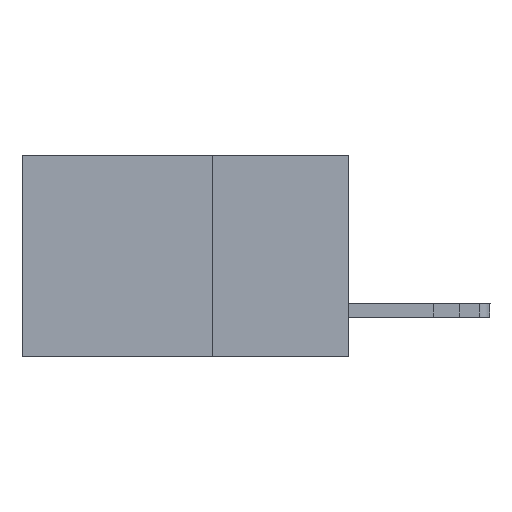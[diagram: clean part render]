
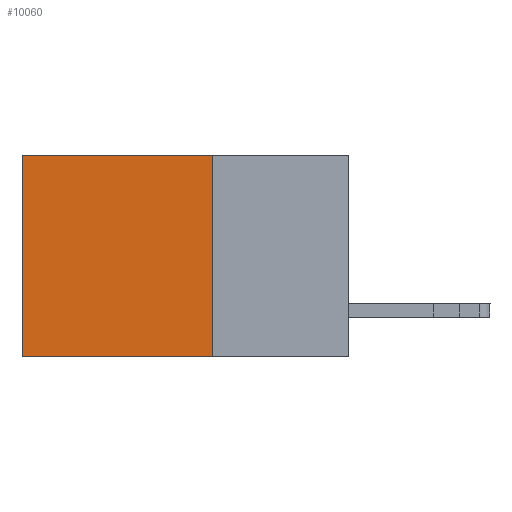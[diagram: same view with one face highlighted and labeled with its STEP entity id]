
A CAD part, left-side view. The second image highlights one B-rep face of the part: STEP entity #10060.
In plain terms, the highlighted planar face has unit normal (-1, 0, 0).
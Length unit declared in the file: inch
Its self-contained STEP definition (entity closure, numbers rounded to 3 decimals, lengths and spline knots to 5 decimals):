
#1041 = ORIENTED_EDGE ( 'NONE', *, *, #10979, .T. ) ;
#1386 = CARTESIAN_POINT ( 'NONE',  ( 0.298, 0.25, 0. ) ) ;
#1926 = CARTESIAN_POINT ( 'NONE',  ( 0.298, 0.25, 0. ) ) ;
#1975 = CARTESIAN_POINT ( 'NONE',  ( 0.298, 0.6, -0.37 ) ) ;
#2164 = CARTESIAN_POINT ( 'NONE',  ( 0.298, 0.25, 0. ) ) ;
#2579 = CARTESIAN_POINT ( 'NONE',  ( 0.298, 0.25, -0.37 ) ) ;
#2600 = CARTESIAN_POINT ( 'NONE',  ( 0.298, 0.6, 0. ) ) ;
#2661 = ORIENTED_EDGE ( 'NONE', *, *, #10180, .F. ) ;
#2903 = ORIENTED_EDGE ( 'NONE', *, *, #3127, .T. ) ;
#2973 = ORIENTED_EDGE ( 'NONE', *, *, #8306, .F. ) ;
#3000 = VECTOR ( 'NONE', #5588, 39.37008 ) ;
#3127 = EDGE_CURVE ( 'NONE', #6355, #10970, #6141, .T. ) ;
#3962 = VECTOR ( 'NONE', #13827, 39.37008 ) ;
#4006 = LINE ( 'NONE', #1386, #9899 ) ;
#4305 = CARTESIAN_POINT ( 'NONE',  ( 0.298, 0.25, -0.37 ) ) ;
#5404 = DIRECTION ( 'NONE',  ( 1., 0., 0. ) ) ;
#5450 = CARTESIAN_POINT ( 'NONE',  ( 0.298, 0.25, 0. ) ) ;
#5588 = DIRECTION ( 'NONE',  ( 0., 1., 0. ) ) ;
#5923 = VERTEX_POINT ( 'NONE', #1975 ) ;
#6002 = LINE ( 'NONE', #4305, #3962 ) ;
#6017 = FACE_OUTER_BOUND ( 'NONE', #13135, .T. ) ;
#6141 = LINE ( 'NONE', #2164, #3000 ) ;
#6233 = DIRECTION ( 'NONE',  ( 0., 0., -1. ) ) ;
#6355 = VERTEX_POINT ( 'NONE', #1926 ) ;
#7403 = CARTESIAN_POINT ( 'NONE',  ( 0.298, 0.6, 0. ) ) ;
#7746 = PLANE ( 'NONE',  #8399 ) ;
#8158 = LINE ( 'NONE', #7403, #8531 ) ;
#8306 = EDGE_CURVE ( 'NONE', #6355, #12272, #4006, .T. ) ;
#8399 = AXIS2_PLACEMENT_3D ( 'NONE', #5450, #5404, #9058 ) ;
#8531 = VECTOR ( 'NONE', #6233, 39.37008 ) ;
#9058 = DIRECTION ( 'NONE',  ( 0., 0., -1. ) ) ;
#9899 = VECTOR ( 'NONE', #13158, 39.37008 ) ;
#10060 = ADVANCED_FACE ( 'NONE', ( #6017 ), #7746, .F. ) ;
#10180 = EDGE_CURVE ( 'NONE', #12272, #5923, #6002, .T. ) ;
#10970 = VERTEX_POINT ( 'NONE', #2600 ) ;
#10979 = EDGE_CURVE ( 'NONE', #10970, #5923, #8158, .T. ) ;
#12272 = VERTEX_POINT ( 'NONE', #2579 ) ;
#13135 = EDGE_LOOP ( 'NONE', ( #1041, #2661, #2973, #2903 ) ) ;
#13158 = DIRECTION ( 'NONE',  ( 0., 0., -1. ) ) ;
#13827 = DIRECTION ( 'NONE',  ( 0., 1., 0. ) ) ;
